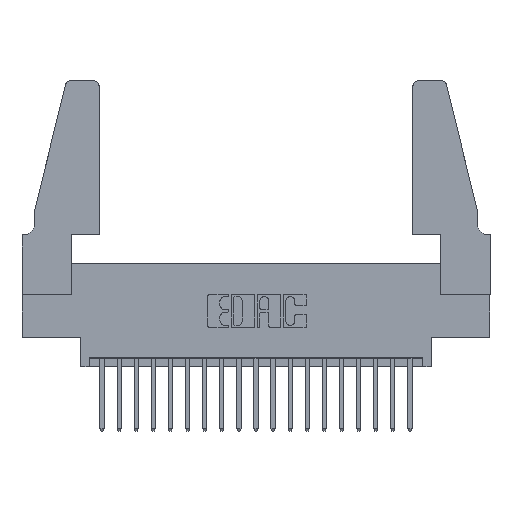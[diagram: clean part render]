
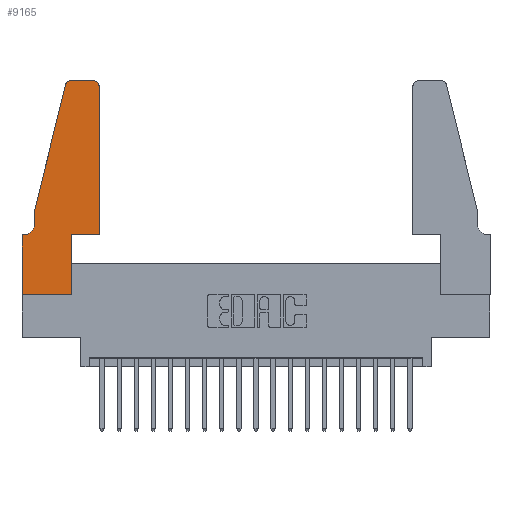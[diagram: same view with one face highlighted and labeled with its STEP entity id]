
A CAD part, top view. The second image highlights one B-rep face of the part: STEP entity #9165.
In plain terms, the highlighted planar face has unit normal (0, 0, 1).
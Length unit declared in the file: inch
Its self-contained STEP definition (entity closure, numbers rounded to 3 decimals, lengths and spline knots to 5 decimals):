
#136 = CIRCLE ( 'NONE', #4819, 0.07 ) ;
#510 = CARTESIAN_POINT ( 'NONE',  ( 0.2865, 0.35, 0.37 ) ) ;
#532 = EDGE_CURVE ( 'NONE', #9195, #4865, #17552, .T. ) ;
#711 = EDGE_LOOP ( 'NONE', ( #1966, #8993, #11387, #2380, #4231, #2618, #4689, #3881, #3445, #9405, #14441, #13798 ) ) ;
#1234 = DIRECTION ( 'NONE',  ( 0., 0., -1. ) ) ;
#1263 = CARTESIAN_POINT ( 'NONE',  ( 0., 0., 0.37 ) ) ;
#1966 = ORIENTED_EDGE ( 'NONE', *, *, #14188, .T. ) ;
#2351 = VERTEX_POINT ( 'NONE', #4292 ) ;
#2370 = VECTOR ( 'NONE', #8534, 39.37008 ) ;
#2380 = ORIENTED_EDGE ( 'NONE', *, *, #16172, .T. ) ;
#2468 = AXIS2_PLACEMENT_3D ( 'NONE', #15903, #4817, #6554 ) ;
#2618 = ORIENTED_EDGE ( 'NONE', *, *, #9557, .T. ) ;
#2887 = EDGE_CURVE ( 'NONE', #18899, #9195, #10712, .T. ) ;
#2964 = DIRECTION ( 'NONE',  ( 0., -1., 0. ) ) ;
#3111 = VERTEX_POINT ( 'NONE', #1263 ) ;
#3445 = ORIENTED_EDGE ( 'NONE', *, *, #18296, .T. ) ;
#3538 = CIRCLE ( 'NONE', #14554, 0.03 ) ;
#3674 = CARTESIAN_POINT ( 'NONE',  ( 0.0755, 0.42, 0.37 ) ) ;
#3725 = CARTESIAN_POINT ( 'NONE',  ( 0.0755, 0.5, 0.37 ) ) ;
#3763 = CARTESIAN_POINT ( 'NONE',  ( 0.0055, 0.35, 0.37 ) ) ;
#3881 = ORIENTED_EDGE ( 'NONE', *, *, #19205, .T. ) ;
#4113 = CARTESIAN_POINT ( 'NONE',  ( 0., 0., 0.37 ) ) ;
#4219 = CARTESIAN_POINT ( 'NONE',  ( 0.2865, 0.35, 0.37 ) ) ;
#4231 = ORIENTED_EDGE ( 'NONE', *, *, #11496, .T. ) ;
#4292 = CARTESIAN_POINT ( 'NONE',  ( 0., 0.35, 0.37 ) ) ;
#4689 = ORIENTED_EDGE ( 'NONE', *, *, #17879, .T. ) ;
#4817 = DIRECTION ( 'NONE',  ( 0., 0., 1. ) ) ;
#4819 = AXIS2_PLACEMENT_3D ( 'NONE', #18480, #1234, #7682 ) ;
#4865 = VERTEX_POINT ( 'NONE', #7769 ) ;
#5256 = DIRECTION ( 'NONE',  ( 0., 1., 0. ) ) ;
#5365 = VECTOR ( 'NONE', #15928, 39.37008 ) ;
#5512 = CARTESIAN_POINT ( 'NONE',  ( 0.284, 1.25, 0.37 ) ) ;
#5655 = EDGE_CURVE ( 'NONE', #4865, #6687, #5917, .T. ) ;
#5721 = DIRECTION ( 'NONE',  ( 1., 0., 0. ) ) ;
#5917 = CIRCLE ( 'NONE', #2468, 0.03 ) ;
#5941 = CARTESIAN_POINT ( 'NONE',  ( 0.284, 1.22, 0.37 ) ) ;
#6296 = LINE ( 'NONE', #15457, #18969 ) ;
#6444 = VECTOR ( 'NONE', #6880, 39.37008 ) ;
#6554 = DIRECTION ( 'NONE',  ( 1., 0., 0. ) ) ;
#6687 = VERTEX_POINT ( 'NONE', #17009 ) ;
#6763 = VERTEX_POINT ( 'NONE', #12799 ) ;
#6880 = DIRECTION ( 'NONE',  ( -1., 0., 0. ) ) ;
#7520 = VECTOR ( 'NONE', #8368, 39.37008 ) ;
#7580 = DIRECTION ( 'NONE',  ( -0.239, -0.971, 0. ) ) ;
#7682 = DIRECTION ( 'NONE',  ( -1., 0., 0. ) ) ;
#7769 = CARTESIAN_POINT ( 'NONE',  ( 0.4505, 1.22, 0.37 ) ) ;
#7944 = LINE ( 'NONE', #11421, #6444 ) ;
#8014 = CARTESIAN_POINT ( 'NONE',  ( 0.4505, 0.35, 0.37 ) ) ;
#8312 = VERTEX_POINT ( 'NONE', #11177 ) ;
#8368 = DIRECTION ( 'NONE',  ( 1., 0., 0. ) ) ;
#8534 = DIRECTION ( 'NONE',  ( 0., -1., 0. ) ) ;
#8993 = ORIENTED_EDGE ( 'NONE', *, *, #12242, .T. ) ;
#9052 = DIRECTION ( 'NONE',  ( 0., 0., 1. ) ) ;
#9115 = DIRECTION ( 'NONE',  ( 1., 0., 0. ) ) ;
#9165 = ADVANCED_FACE ( 'NONE', ( #15434 ), #18459, .T. ) ;
#9192 = VECTOR ( 'NONE', #5721, 39.37008 ) ;
#9195 = VERTEX_POINT ( 'NONE', #8014 ) ;
#9296 = LINE ( 'NONE', #16921, #10747 ) ;
#9353 = LINE ( 'NONE', #15651, #5365 ) ;
#9405 = ORIENTED_EDGE ( 'NONE', *, *, #2887, .T. ) ;
#9557 = EDGE_CURVE ( 'NONE', #13613, #2351, #9353, .T. ) ;
#9883 = DIRECTION ( 'NONE',  ( 0., 0., 1. ) ) ;
#10712 = LINE ( 'NONE', #14346, #7520 ) ;
#10747 = VECTOR ( 'NONE', #7580, 39.37008 ) ;
#11177 = CARTESIAN_POINT ( 'NONE',  ( 0.2865, 0., 0.37 ) ) ;
#11387 = ORIENTED_EDGE ( 'NONE', *, *, #17086, .T. ) ;
#11421 = CARTESIAN_POINT ( 'NONE',  ( 0.2605, 1.25, 0.37 ) ) ;
#11496 = EDGE_CURVE ( 'NONE', #17398, #13613, #136, .T. ) ;
#11800 = CARTESIAN_POINT ( 'NONE',  ( 0.25487, 1.22718, 0.37 ) ) ;
#11811 = VERTEX_POINT ( 'NONE', #11800 ) ;
#12242 = EDGE_CURVE ( 'NONE', #16856, #11811, #3538, .T. ) ;
#12799 = CARTESIAN_POINT ( 'NONE',  ( 0.0755, 0.5, 0.37 ) ) ;
#13025 = CARTESIAN_POINT ( 'NONE',  ( 0.4505, 0.35, 0.37 ) ) ;
#13465 = LINE ( 'NONE', #3725, #2370 ) ;
#13613 = VERTEX_POINT ( 'NONE', #3763 ) ;
#13669 = CARTESIAN_POINT ( 'NONE',  ( 0., 0.35, 0.37 ) ) ;
#13798 = ORIENTED_EDGE ( 'NONE', *, *, #5655, .T. ) ;
#14188 = EDGE_CURVE ( 'NONE', #6687, #16856, #7944, .T. ) ;
#14346 = CARTESIAN_POINT ( 'NONE',  ( 0.4505, 0.35, 0.37 ) ) ;
#14441 = ORIENTED_EDGE ( 'NONE', *, *, #532, .T. ) ;
#14554 = AXIS2_PLACEMENT_3D ( 'NONE', #5941, #9883, #17665 ) ;
#14980 = DIRECTION ( 'NONE',  ( 0., 1., 0. ) ) ;
#15434 = FACE_OUTER_BOUND ( 'NONE', #711, .T. ) ;
#15457 = CARTESIAN_POINT ( 'NONE',  ( 0., 0., 0.37 ) ) ;
#15651 = CARTESIAN_POINT ( 'NONE',  ( 0.0755, 0.35, 0.37 ) ) ;
#15903 = CARTESIAN_POINT ( 'NONE',  ( 0.4205, 1.22, 0.37 ) ) ;
#15928 = DIRECTION ( 'NONE',  ( -1., 0., 0. ) ) ;
#16172 = EDGE_CURVE ( 'NONE', #6763, #17398, #13465, .T. ) ;
#16765 = VECTOR ( 'NONE', #14980, 39.37008 ) ;
#16856 = VERTEX_POINT ( 'NONE', #5512 ) ;
#16921 = CARTESIAN_POINT ( 'NONE',  ( 0.0755, 0.5, 0.37 ) ) ;
#17009 = CARTESIAN_POINT ( 'NONE',  ( 0.4205, 1.25, 0.37 ) ) ;
#17086 = EDGE_CURVE ( 'NONE', #11811, #6763, #9296, .T. ) ;
#17398 = VERTEX_POINT ( 'NONE', #3674 ) ;
#17552 = LINE ( 'NONE', #13025, #18019 ) ;
#17665 = DIRECTION ( 'NONE',  ( 1., 0., 0. ) ) ;
#17879 = EDGE_CURVE ( 'NONE', #2351, #3111, #6296, .T. ) ;
#18019 = VECTOR ( 'NONE', #5256, 39.37008 ) ;
#18213 = LINE ( 'NONE', #4219, #16765 ) ;
#18296 = EDGE_CURVE ( 'NONE', #8312, #18899, #18213, .T. ) ;
#18459 = PLANE ( 'NONE',  #18667 ) ;
#18480 = CARTESIAN_POINT ( 'NONE',  ( 0.0055, 0.42, 0.37 ) ) ;
#18667 = AXIS2_PLACEMENT_3D ( 'NONE', #13669, #9052, #9115 ) ;
#18899 = VERTEX_POINT ( 'NONE', #510 ) ;
#18969 = VECTOR ( 'NONE', #2964, 39.37008 ) ;
#19205 = EDGE_CURVE ( 'NONE', #3111, #8312, #20157, .T. ) ;
#20157 = LINE ( 'NONE', #4113, #9192 ) ;
